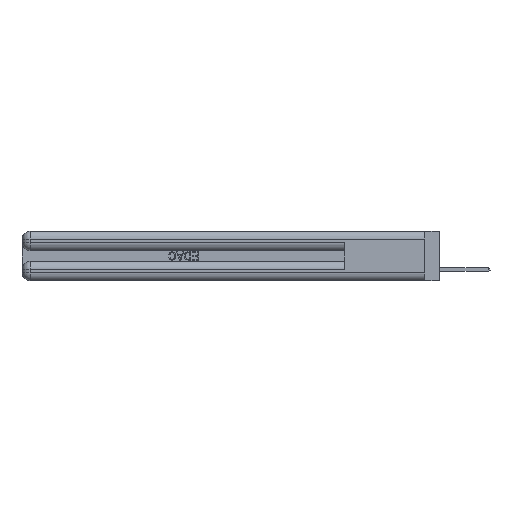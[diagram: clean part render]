
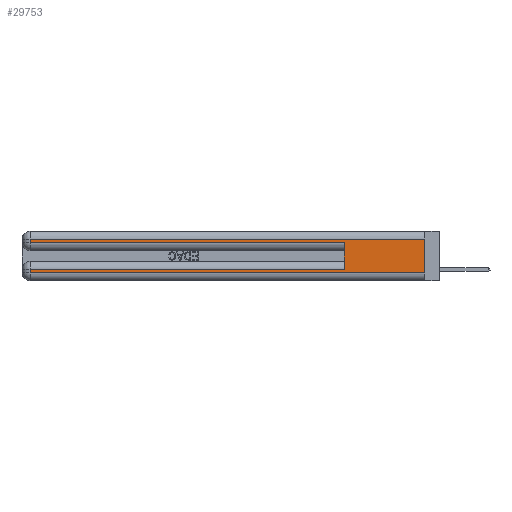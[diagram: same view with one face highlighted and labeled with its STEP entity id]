
A CAD part, left-side view. The second image highlights one B-rep face of the part: STEP entity #29753.
In plain terms, the highlighted planar face has unit normal (-1, 0, 0).
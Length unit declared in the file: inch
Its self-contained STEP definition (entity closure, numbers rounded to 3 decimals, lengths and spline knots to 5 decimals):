
#1443 = VERTEX_POINT ( 'NONE', #19626 ) ;
#2886 = LINE ( 'NONE', #50428, #13884 ) ;
#3208 = EDGE_CURVE ( 'NONE', #21332, #39179, #44439, .T. ) ;
#3233 = CARTESIAN_POINT ( 'NONE',  ( 0., 0., 0.37 ) ) ;
#3761 = DIRECTION ( 'NONE',  ( 1., 0., 0. ) ) ;
#4107 = LINE ( 'NONE', #39293, #17766 ) ;
#4324 = EDGE_CURVE ( 'NONE', #21332, #49997, #27540, .T. ) ;
#5376 = VECTOR ( 'NONE', #28593, 39.37008 ) ;
#5517 = VECTOR ( 'NONE', #9961, 39.37008 ) ;
#6993 = CARTESIAN_POINT ( 'NONE',  ( 0., 0.6, 0.285 ) ) ;
#7776 = EDGE_LOOP ( 'NONE', ( #30394, #14083, #48570, #45649, #43279, #8844, #11061, #25278 ) ) ;
#8763 = VERTEX_POINT ( 'NONE', #10432 ) ;
#8844 = ORIENTED_EDGE ( 'NONE', *, *, #4324, .T. ) ;
#9961 = DIRECTION ( 'NONE',  ( 0., 0., 1. ) ) ;
#10432 = CARTESIAN_POINT ( 'NONE',  ( 0., 2.94, 0.06 ) ) ;
#10458 = CARTESIAN_POINT ( 'NONE',  ( 0., 0., 0.06 ) ) ;
#10556 = FACE_OUTER_BOUND ( 'NONE', #7776, .T. ) ;
#10792 = CARTESIAN_POINT ( 'NONE',  ( 0., 0., 0.085 ) ) ;
#11061 = ORIENTED_EDGE ( 'NONE', *, *, #29602, .T. ) ;
#11734 = DIRECTION ( 'NONE',  ( 0., 0., -1. ) ) ;
#13884 = VECTOR ( 'NONE', #21657, 39.37008 ) ;
#14083 = ORIENTED_EDGE ( 'NONE', *, *, #43448, .T. ) ;
#15446 = EDGE_CURVE ( 'NONE', #46645, #1443, #18510, .T. ) ;
#16708 = CARTESIAN_POINT ( 'NONE',  ( 0., 0., 0.06 ) ) ;
#17326 = AXIS2_PLACEMENT_3D ( 'NONE', #3233, #3761, #11734 ) ;
#17766 = VECTOR ( 'NONE', #39660, 39.37008 ) ;
#18331 = EDGE_CURVE ( 'NONE', #8763, #28200, #31159, .T. ) ;
#18461 = VECTOR ( 'NONE', #45919, 39.37008 ) ;
#18510 = LINE ( 'NONE', #34329, #49590 ) ;
#19626 = CARTESIAN_POINT ( 'NONE',  ( 0., 2.94, 0.285 ) ) ;
#21241 = DIRECTION ( 'NONE',  ( 0., -1., 0. ) ) ;
#21332 = VERTEX_POINT ( 'NONE', #34531 ) ;
#21657 = DIRECTION ( 'NONE',  ( 0., 0., -1. ) ) ;
#23362 = DIRECTION ( 'NONE',  ( 0., 1., 0. ) ) ;
#24073 = CARTESIAN_POINT ( 'NONE',  ( 0., 0., 0.31 ) ) ;
#25278 = ORIENTED_EDGE ( 'NONE', *, *, #18331, .T. ) ;
#26643 = LINE ( 'NONE', #48531, #5376 ) ;
#27540 = LINE ( 'NONE', #10792, #30124 ) ;
#28200 = VERTEX_POINT ( 'NONE', #10458 ) ;
#28433 = PLANE ( 'NONE',  #17326 ) ;
#28593 = DIRECTION ( 'NONE',  ( 0., 1., 0. ) ) ;
#29106 = EDGE_CURVE ( 'NONE', #35715, #28200, #2886, .T. ) ;
#29602 = EDGE_CURVE ( 'NONE', #49997, #8763, #4107, .T. ) ;
#29753 = ADVANCED_FACE ( 'NONE', ( #10556 ), #28433, .F. ) ;
#29861 = VECTOR ( 'NONE', #21241, 39.37008 ) ;
#30124 = VECTOR ( 'NONE', #23362, 39.37008 ) ;
#30394 = ORIENTED_EDGE ( 'NONE', *, *, #29106, .F. ) ;
#31159 = LINE ( 'NONE', #16708, #29861 ) ;
#31940 = CARTESIAN_POINT ( 'NONE',  ( 0., 2.94, 0.085 ) ) ;
#34329 = CARTESIAN_POINT ( 'NONE',  ( 0., 2.94, 0.37 ) ) ;
#34508 = DIRECTION ( 'NONE',  ( 0., 0., -1. ) ) ;
#34531 = CARTESIAN_POINT ( 'NONE',  ( 0., 0.6, 0.085 ) ) ;
#35715 = VERTEX_POINT ( 'NONE', #24073 ) ;
#36541 = LINE ( 'NONE', #50256, #18461 ) ;
#39179 = VERTEX_POINT ( 'NONE', #6993 ) ;
#39293 = CARTESIAN_POINT ( 'NONE',  ( 0., 2.94, 0.37 ) ) ;
#39660 = DIRECTION ( 'NONE',  ( 0., 0., -1. ) ) ;
#41348 = CARTESIAN_POINT ( 'NONE',  ( 0., 2.94, 0.31 ) ) ;
#43279 = ORIENTED_EDGE ( 'NONE', *, *, #3208, .F. ) ;
#43448 = EDGE_CURVE ( 'NONE', #35715, #46645, #26643, .T. ) ;
#44439 = LINE ( 'NONE', #46837, #5517 ) ;
#45649 = ORIENTED_EDGE ( 'NONE', *, *, #49540, .T. ) ;
#45919 = DIRECTION ( 'NONE',  ( 0., -1., 0. ) ) ;
#46645 = VERTEX_POINT ( 'NONE', #41348 ) ;
#46837 = CARTESIAN_POINT ( 'NONE',  ( 0., 0.6, 0.145 ) ) ;
#48531 = CARTESIAN_POINT ( 'NONE',  ( 0., 0., 0.31 ) ) ;
#48570 = ORIENTED_EDGE ( 'NONE', *, *, #15446, .T. ) ;
#49540 = EDGE_CURVE ( 'NONE', #1443, #39179, #36541, .T. ) ;
#49590 = VECTOR ( 'NONE', #34508, 39.37008 ) ;
#49997 = VERTEX_POINT ( 'NONE', #31940 ) ;
#50256 = CARTESIAN_POINT ( 'NONE',  ( 0., 0., 0.285 ) ) ;
#50428 = CARTESIAN_POINT ( 'NONE',  ( 0., 0., 0.37 ) ) ;
